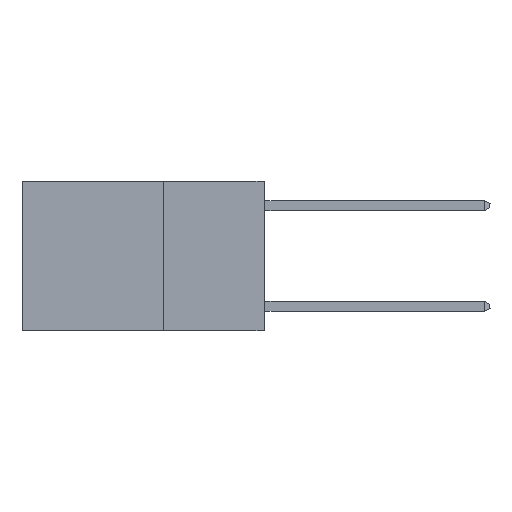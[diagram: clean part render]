
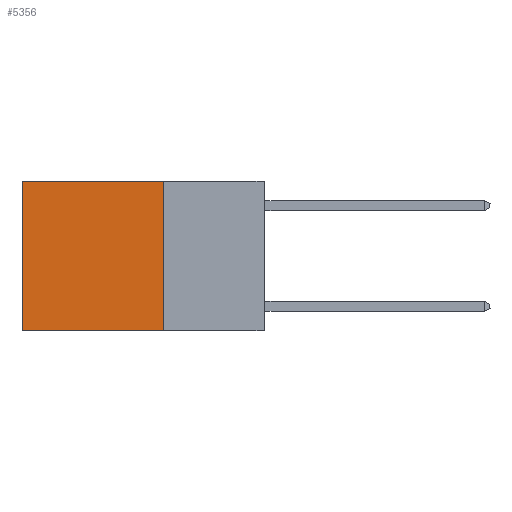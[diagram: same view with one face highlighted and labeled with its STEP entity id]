
A CAD part, left-side view. The second image highlights one B-rep face of the part: STEP entity #5356.
In plain terms, the highlighted planar face has unit normal (-1, 0, 0).
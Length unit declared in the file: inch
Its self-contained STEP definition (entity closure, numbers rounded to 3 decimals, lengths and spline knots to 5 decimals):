
#485 = DIRECTION ( 'NONE',  ( 0., 0., -1. ) ) ;
#584 = FACE_OUTER_BOUND ( 'NONE', #16486, .T. ) ;
#967 = DIRECTION ( 'NONE',  ( 0., 0., -1. ) ) ;
#1176 = EDGE_CURVE ( 'NONE', #12787, #14489, #4898, .T. ) ;
#1758 = DIRECTION ( 'NONE',  ( 0., 0., -1. ) ) ;
#1878 = CARTESIAN_POINT ( 'NONE',  ( 0.2625, 0.25, -0.37 ) ) ;
#1906 = PLANE ( 'NONE',  #11015 ) ;
#2912 = LINE ( 'NONE', #11776, #9319 ) ;
#4776 = LINE ( 'NONE', #1878, #11596 ) ;
#4898 = LINE ( 'NONE', #10813, #6348 ) ;
#5356 = ADVANCED_FACE ( 'NONE', ( #584 ), #1906, .F. ) ;
#6348 = VECTOR ( 'NONE', #15247, 39.37008 ) ;
#7809 = CARTESIAN_POINT ( 'NONE',  ( 0.2625, 0.25, 0. ) ) ;
#9256 = ORIENTED_EDGE ( 'NONE', *, *, #13788, .F. ) ;
#9319 = VECTOR ( 'NONE', #1758, 39.37008 ) ;
#9774 = CARTESIAN_POINT ( 'NONE',  ( 0.2625, 0.25, 0. ) ) ;
#10813 = CARTESIAN_POINT ( 'NONE',  ( 0.2625, 0.25, 0. ) ) ;
#11001 = CARTESIAN_POINT ( 'NONE',  ( 0.2625, 0.6, 0. ) ) ;
#11015 = AXIS2_PLACEMENT_3D ( 'NONE', #7809, #13712, #485 ) ;
#11596 = VECTOR ( 'NONE', #16861, 39.37008 ) ;
#11776 = CARTESIAN_POINT ( 'NONE',  ( 0.2625, 0.6, 0. ) ) ;
#12654 = ORIENTED_EDGE ( 'NONE', *, *, #18726, .T. ) ;
#12787 = VERTEX_POINT ( 'NONE', #15258 ) ;
#13190 = CARTESIAN_POINT ( 'NONE',  ( 0.2625, 0.6, -0.37 ) ) ;
#13418 = VECTOR ( 'NONE', #967, 39.37008 ) ;
#13596 = ORIENTED_EDGE ( 'NONE', *, *, #14002, .F. ) ;
#13712 = DIRECTION ( 'NONE',  ( 1., 0., 0. ) ) ;
#13788 = EDGE_CURVE ( 'NONE', #17123, #15047, #4776, .T. ) ;
#14002 = EDGE_CURVE ( 'NONE', #12787, #17123, #18747, .T. ) ;
#14489 = VERTEX_POINT ( 'NONE', #11001 ) ;
#15047 = VERTEX_POINT ( 'NONE', #13190 ) ;
#15247 = DIRECTION ( 'NONE',  ( 0., 1., 0. ) ) ;
#15258 = CARTESIAN_POINT ( 'NONE',  ( 0.2625, 0.25, 0. ) ) ;
#15944 = CARTESIAN_POINT ( 'NONE',  ( 0.2625, 0.25, -0.37 ) ) ;
#16486 = EDGE_LOOP ( 'NONE', ( #12654, #9256, #13596, #17407 ) ) ;
#16861 = DIRECTION ( 'NONE',  ( 0., 1., 0. ) ) ;
#17123 = VERTEX_POINT ( 'NONE', #15944 ) ;
#17407 = ORIENTED_EDGE ( 'NONE', *, *, #1176, .T. ) ;
#18726 = EDGE_CURVE ( 'NONE', #14489, #15047, #2912, .T. ) ;
#18747 = LINE ( 'NONE', #9774, #13418 ) ;
